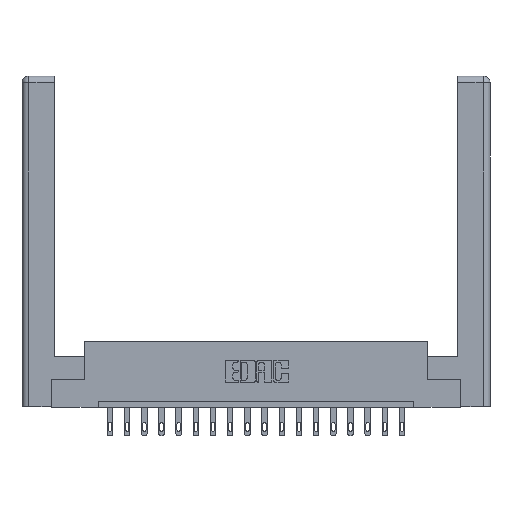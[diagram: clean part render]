
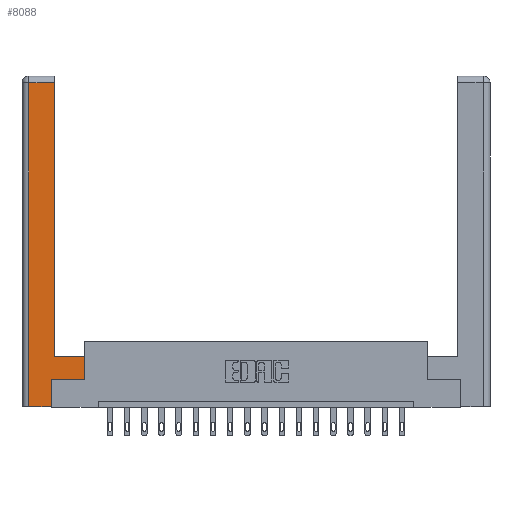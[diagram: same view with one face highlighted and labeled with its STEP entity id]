
A CAD part, top view. The second image highlights one B-rep face of the part: STEP entity #8088.
In plain terms, the highlighted planar face has unit normal (0, 0, 1).
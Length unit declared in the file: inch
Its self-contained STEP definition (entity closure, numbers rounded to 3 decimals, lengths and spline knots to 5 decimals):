
#184 = VECTOR ( 'NONE', #2075, 39.37008 ) ;
#653 = VERTEX_POINT ( 'NONE', #4959 ) ;
#758 = DIRECTION ( 'NONE',  ( 0., -1., 0. ) ) ;
#891 = ORIENTED_EDGE ( 'NONE', *, *, #9016, .T. ) ;
#1103 = CARTESIAN_POINT ( 'NONE',  ( 0.0615, 0., 0. ) ) ;
#1200 = VECTOR ( 'NONE', #18394, 39.37008 ) ;
#1966 = CARTESIAN_POINT ( 'NONE',  ( 0.0615, 2.94, 0. ) ) ;
#2023 = LINE ( 'NONE', #9574, #5236 ) ;
#2075 = DIRECTION ( 'NONE',  ( 0., 1., 0. ) ) ;
#2293 = VERTEX_POINT ( 'NONE', #1103 ) ;
#3301 = EDGE_CURVE ( 'NONE', #2293, #11636, #3739, .T. ) ;
#3484 = VERTEX_POINT ( 'NONE', #1966 ) ;
#3581 = VERTEX_POINT ( 'NONE', #5549 ) ;
#3658 = CARTESIAN_POINT ( 'NONE',  ( 0.295, 3., 0. ) ) ;
#3739 = LINE ( 'NONE', #12890, #6033 ) ;
#4221 = DIRECTION ( 'NONE',  ( 1., 0., 0. ) ) ;
#4655 = ORIENTED_EDGE ( 'NONE', *, *, #6081, .T. ) ;
#4779 = LINE ( 'NONE', #7294, #10786 ) ;
#4905 = ORIENTED_EDGE ( 'NONE', *, *, #14952, .T. ) ;
#4920 = ORIENTED_EDGE ( 'NONE', *, *, #10244, .T. ) ;
#4959 = CARTESIAN_POINT ( 'NONE',  ( 0.565, 0.245, 0. ) ) ;
#5219 = CARTESIAN_POINT ( 'NONE',  ( 0.295, 2.94, 0. ) ) ;
#5236 = VECTOR ( 'NONE', #758, 39.37008 ) ;
#5309 = CARTESIAN_POINT ( 'NONE',  ( 0., 0., 0. ) ) ;
#5319 = ORIENTED_EDGE ( 'NONE', *, *, #12035, .T. ) ;
#5365 = CARTESIAN_POINT ( 'NONE',  ( 0.565, 0.245, 0. ) ) ;
#5371 = DIRECTION ( 'NONE',  ( 0., 0., -1. ) ) ;
#5549 = CARTESIAN_POINT ( 'NONE',  ( 0.295, 0.45, 0. ) ) ;
#6033 = VECTOR ( 'NONE', #4221, 39.37008 ) ;
#6081 = EDGE_CURVE ( 'NONE', #11636, #15059, #10633, .T. ) ;
#6807 = VECTOR ( 'NONE', #9739, 39.37008 ) ;
#7241 = EDGE_LOOP ( 'NONE', ( #7693, #10762, #5319, #9699, #4655, #4920, #891, #4905 ) ) ;
#7294 = CARTESIAN_POINT ( 'NONE',  ( 0.0615, 2.94, 0. ) ) ;
#7648 = VECTOR ( 'NONE', #18864, 39.37008 ) ;
#7693 = ORIENTED_EDGE ( 'NONE', *, *, #15061, .T. ) ;
#8088 = ADVANCED_FACE ( 'NONE', ( #16985 ), #17005, .F. ) ;
#8832 = EDGE_CURVE ( 'NONE', #9786, #3484, #4779, .T. ) ;
#9016 = EDGE_CURVE ( 'NONE', #653, #12225, #14961, .T. ) ;
#9574 = CARTESIAN_POINT ( 'NONE',  ( 0.0615, 0., 0. ) ) ;
#9699 = ORIENTED_EDGE ( 'NONE', *, *, #3301, .T. ) ;
#9739 = DIRECTION ( 'NONE',  ( 1., 0., 0. ) ) ;
#9786 = VERTEX_POINT ( 'NONE', #5219 ) ;
#9944 = LINE ( 'NONE', #3658, #1200 ) ;
#9966 = LINE ( 'NONE', #12893, #10198 ) ;
#10198 = VECTOR ( 'NONE', #17283, 39.37008 ) ;
#10244 = EDGE_CURVE ( 'NONE', #15059, #653, #16266, .T. ) ;
#10633 = LINE ( 'NONE', #14550, #7648 ) ;
#10762 = ORIENTED_EDGE ( 'NONE', *, *, #8832, .T. ) ;
#10786 = VECTOR ( 'NONE', #17389, 39.37008 ) ;
#11008 = CARTESIAN_POINT ( 'NONE',  ( 0.265, 0.245, 0. ) ) ;
#11636 = VERTEX_POINT ( 'NONE', #17466 ) ;
#12035 = EDGE_CURVE ( 'NONE', #3484, #2293, #2023, .T. ) ;
#12225 = VERTEX_POINT ( 'NONE', #18091 ) ;
#12318 = CARTESIAN_POINT ( 'NONE',  ( 0.565, 0.45, 0. ) ) ;
#12890 = CARTESIAN_POINT ( 'NONE',  ( 0.265, 0., 0. ) ) ;
#12893 = CARTESIAN_POINT ( 'NONE',  ( 0.295, 0.45, 0. ) ) ;
#13935 = AXIS2_PLACEMENT_3D ( 'NONE', #5309, #5371, #17200 ) ;
#14550 = CARTESIAN_POINT ( 'NONE',  ( 0.265, 0.245, 0. ) ) ;
#14952 = EDGE_CURVE ( 'NONE', #12225, #3581, #9966, .T. ) ;
#14961 = LINE ( 'NONE', #12318, #184 ) ;
#15059 = VERTEX_POINT ( 'NONE', #11008 ) ;
#15061 = EDGE_CURVE ( 'NONE', #3581, #9786, #9944, .T. ) ;
#16266 = LINE ( 'NONE', #5365, #6807 ) ;
#16985 = FACE_OUTER_BOUND ( 'NONE', #7241, .T. ) ;
#17005 = PLANE ( 'NONE',  #13935 ) ;
#17200 = DIRECTION ( 'NONE',  ( -1., 0., 0. ) ) ;
#17283 = DIRECTION ( 'NONE',  ( -1., 0., 0. ) ) ;
#17389 = DIRECTION ( 'NONE',  ( -1., 0., 0. ) ) ;
#17466 = CARTESIAN_POINT ( 'NONE',  ( 0.265, 0., 0. ) ) ;
#18091 = CARTESIAN_POINT ( 'NONE',  ( 0.565, 0.45, 0. ) ) ;
#18394 = DIRECTION ( 'NONE',  ( 0., 1., 0. ) ) ;
#18864 = DIRECTION ( 'NONE',  ( 0., 1., 0. ) ) ;
